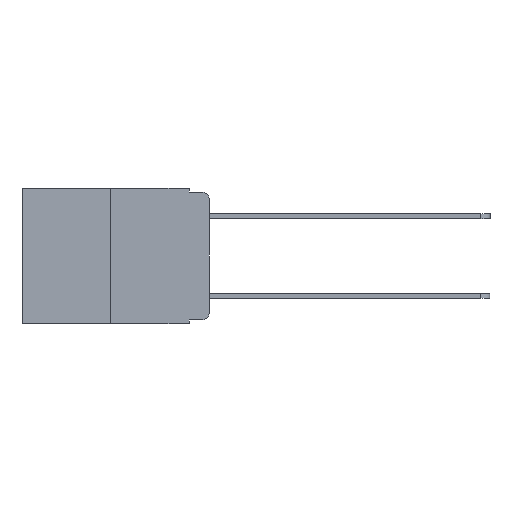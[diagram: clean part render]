
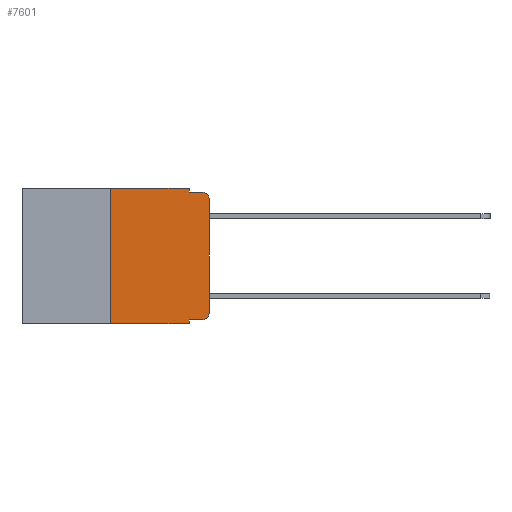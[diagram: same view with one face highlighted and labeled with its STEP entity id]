
A CAD part, left-side view. The second image highlights one B-rep face of the part: STEP entity #7601.
In plain terms, the highlighted planar face has unit normal (-1, 0, 0).
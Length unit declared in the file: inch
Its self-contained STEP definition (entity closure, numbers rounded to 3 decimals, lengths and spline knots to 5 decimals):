
#257 = DIRECTION ( 'NONE',  ( 0., 0., -1. ) ) ;
#444 = CARTESIAN_POINT ( 'NONE',  ( 0., 0.051, 0. ) ) ;
#469 = CARTESIAN_POINT ( 'NONE',  ( 0., 0.02, -0.03 ) ) ;
#564 = DIRECTION ( 'NONE',  ( 0., 0., 1. ) ) ;
#603 = EDGE_LOOP ( 'NONE', ( #2280, #3390, #2798, #3340, #3181, #6354, #5258, #5066, #3311, #3193 ) ) ;
#745 = CARTESIAN_POINT ( 'NONE',  ( 0., 0.473, 0. ) ) ;
#883 = LINE ( 'NONE', #7780, #9320 ) ;
#887 = LINE ( 'NONE', #5351, #2992 ) ;
#957 = LINE ( 'NONE', #8871, #5024 ) ;
#1070 = DIRECTION ( 'NONE',  ( 1., 0., 0. ) ) ;
#1146 = VERTEX_POINT ( 'NONE', #3948 ) ;
#1339 = CARTESIAN_POINT ( 'NONE',  ( 0., 0.25, 0. ) ) ;
#1446 = DIRECTION ( 'NONE',  ( 0., 0., -1. ) ) ;
#1562 = VERTEX_POINT ( 'NONE', #6248 ) ;
#1615 = PLANE ( 'NONE',  #7583 ) ;
#1690 = LINE ( 'NONE', #1339, #6672 ) ;
#1775 = LINE ( 'NONE', #8560, #7826 ) ;
#2101 = EDGE_CURVE ( 'NONE', #9785, #4088, #957, .T. ) ;
#2171 = DIRECTION ( 'NONE',  ( 0., 0., 1. ) ) ;
#2195 = CARTESIAN_POINT ( 'NONE',  ( 0., 0., -0.03 ) ) ;
#2280 = ORIENTED_EDGE ( 'NONE', *, *, #8118, .T. ) ;
#2453 = EDGE_CURVE ( 'NONE', #1146, #6882, #4345, .T. ) ;
#2470 = LINE ( 'NONE', #444, #4443 ) ;
#2668 = EDGE_CURVE ( 'NONE', #3012, #8615, #1690, .T. ) ;
#2798 = ORIENTED_EDGE ( 'NONE', *, *, #6581, .F. ) ;
#2875 = CIRCLE ( 'NONE', #6821, 0.02 ) ;
#2992 = VECTOR ( 'NONE', #4484, 39.37008 ) ;
#3012 = VERTEX_POINT ( 'NONE', #5206 ) ;
#3153 = CARTESIAN_POINT ( 'NONE',  ( 0., 0.25, 0. ) ) ;
#3181 = ORIENTED_EDGE ( 'NONE', *, *, #9542, .F. ) ;
#3193 = ORIENTED_EDGE ( 'NONE', *, *, #2453, .T. ) ;
#3259 = VERTEX_POINT ( 'NONE', #2195 ) ;
#3311 = ORIENTED_EDGE ( 'NONE', *, *, #7426, .T. ) ;
#3340 = ORIENTED_EDGE ( 'NONE', *, *, #2101, .F. ) ;
#3390 = ORIENTED_EDGE ( 'NONE', *, *, #8621, .T. ) ;
#3798 = CARTESIAN_POINT ( 'NONE',  ( 0., 0.02, -0.313 ) ) ;
#3948 = CARTESIAN_POINT ( 'NONE',  ( 0., 0.02, -0.333 ) ) ;
#4088 = VERTEX_POINT ( 'NONE', #7272 ) ;
#4233 = DIRECTION ( 'NONE',  ( 0., -1., 0. ) ) ;
#4345 = CIRCLE ( 'NONE', #9114, 0.02 ) ;
#4443 = VECTOR ( 'NONE', #5303, 39.37008 ) ;
#4460 = VECTOR ( 'NONE', #564, 39.37008 ) ;
#4484 = DIRECTION ( 'NONE',  ( 0., -1., 0. ) ) ;
#4648 = VERTEX_POINT ( 'NONE', #9002 ) ;
#5024 = VECTOR ( 'NONE', #8795, 39.37008 ) ;
#5041 = VERTEX_POINT ( 'NONE', #5846 ) ;
#5066 = ORIENTED_EDGE ( 'NONE', *, *, #5293, .F. ) ;
#5206 = CARTESIAN_POINT ( 'NONE',  ( 0., 0.25, -0.343 ) ) ;
#5258 = ORIENTED_EDGE ( 'NONE', *, *, #6526, .T. ) ;
#5293 = EDGE_CURVE ( 'NONE', #5041, #4648, #2470, .T. ) ;
#5303 = DIRECTION ( 'NONE',  ( 0., 0., -1. ) ) ;
#5351 = CARTESIAN_POINT ( 'NONE',  ( 0., 0.473, 0. ) ) ;
#5399 = CARTESIAN_POINT ( 'NONE',  ( 0., 0.051, -0.333 ) ) ;
#5817 = DIRECTION ( 'NONE',  ( 0., 0., -1. ) ) ;
#5840 = DIRECTION ( 'NONE',  ( -1., 0., 0. ) ) ;
#5846 = CARTESIAN_POINT ( 'NONE',  ( 0., 0.051, -0.333 ) ) ;
#6248 = CARTESIAN_POINT ( 'NONE',  ( 0., 0.02, -0.01 ) ) ;
#6354 = ORIENTED_EDGE ( 'NONE', *, *, #2668, .F. ) ;
#6507 = DIRECTION ( 'NONE',  ( -1., 0., 0. ) ) ;
#6526 = EDGE_CURVE ( 'NONE', #3012, #4648, #1775, .T. ) ;
#6581 = EDGE_CURVE ( 'NONE', #4088, #1562, #883, .T. ) ;
#6618 = CARTESIAN_POINT ( 'NONE',  ( 0., 0.051, 0. ) ) ;
#6672 = VECTOR ( 'NONE', #2171, 39.37008 ) ;
#6794 = DIRECTION ( 'NONE',  ( 0., -1., 0. ) ) ;
#6821 = AXIS2_PLACEMENT_3D ( 'NONE', #469, #6507, #1446 ) ;
#6882 = VERTEX_POINT ( 'NONE', #10000 ) ;
#6987 = VECTOR ( 'NONE', #4233, 39.37008 ) ;
#7216 = LINE ( 'NONE', #5399, #6987 ) ;
#7272 = CARTESIAN_POINT ( 'NONE',  ( 0., 0.051, -0.01 ) ) ;
#7426 = EDGE_CURVE ( 'NONE', #5041, #1146, #7216, .T. ) ;
#7583 = AXIS2_PLACEMENT_3D ( 'NONE', #745, #1070, #257 ) ;
#7601 = ADVANCED_FACE ( 'NONE', ( #9313 ), #1615, .F. ) ;
#7780 = CARTESIAN_POINT ( 'NONE',  ( 0., 0.051, -0.01 ) ) ;
#7826 = VECTOR ( 'NONE', #8479, 39.37008 ) ;
#8118 = EDGE_CURVE ( 'NONE', #6882, #3259, #8679, .T. ) ;
#8479 = DIRECTION ( 'NONE',  ( 0., -1., 0. ) ) ;
#8560 = CARTESIAN_POINT ( 'NONE',  ( 0., 0.473, -0.343 ) ) ;
#8615 = VERTEX_POINT ( 'NONE', #3153 ) ;
#8621 = EDGE_CURVE ( 'NONE', #3259, #1562, #2875, .T. ) ;
#8679 = LINE ( 'NONE', #10317, #4460 ) ;
#8795 = DIRECTION ( 'NONE',  ( 0., 0., -1. ) ) ;
#8871 = CARTESIAN_POINT ( 'NONE',  ( 0., 0.051, 0. ) ) ;
#9002 = CARTESIAN_POINT ( 'NONE',  ( 0., 0.051, -0.343 ) ) ;
#9114 = AXIS2_PLACEMENT_3D ( 'NONE', #3798, #5840, #5817 ) ;
#9313 = FACE_OUTER_BOUND ( 'NONE', #603, .T. ) ;
#9320 = VECTOR ( 'NONE', #6794, 39.37008 ) ;
#9542 = EDGE_CURVE ( 'NONE', #8615, #9785, #887, .T. ) ;
#9785 = VERTEX_POINT ( 'NONE', #6618 ) ;
#10000 = CARTESIAN_POINT ( 'NONE',  ( 0., 0., -0.313 ) ) ;
#10317 = CARTESIAN_POINT ( 'NONE',  ( 0., 0., 0. ) ) ;
